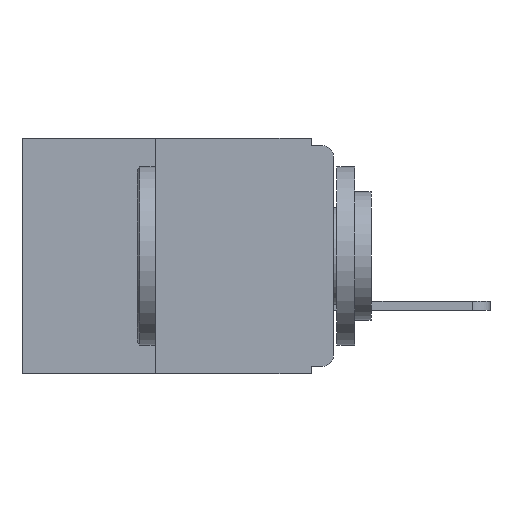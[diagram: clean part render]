
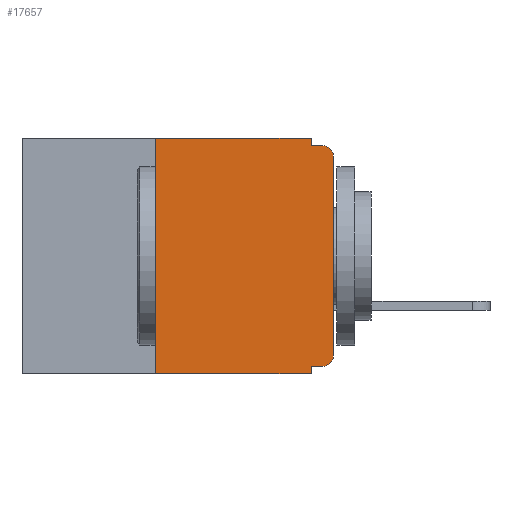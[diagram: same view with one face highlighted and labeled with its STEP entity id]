
A CAD part, left-side view. The second image highlights one B-rep face of the part: STEP entity #17657.
In plain terms, the highlighted planar face has unit normal (-1, 0, 0).
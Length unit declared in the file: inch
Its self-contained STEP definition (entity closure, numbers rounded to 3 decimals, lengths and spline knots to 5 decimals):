
#217 = CIRCLE ( 'NONE', #12686, 0.015 ) ;
#681 = FACE_OUTER_BOUND ( 'NONE', #4384, .T. ) ;
#811 = CARTESIAN_POINT ( 'NONE',  ( 0., 0., -0.32 ) ) ;
#814 = LINE ( 'NONE', #18996, #882 ) ;
#882 = VECTOR ( 'NONE', #18919, 39.37008 ) ;
#887 = VECTOR ( 'NONE', #4522, 39.37008 ) ;
#909 = LINE ( 'NONE', #4687, #887 ) ;
#1333 = DIRECTION ( 'NONE',  ( 0., 1., 0. ) ) ;
#2322 = DIRECTION ( 'NONE',  ( 0., 0., -1. ) ) ;
#2346 = VERTEX_POINT ( 'NONE', #6631 ) ;
#2395 = DIRECTION ( 'NONE',  ( -1., 0., 0. ) ) ;
#2806 = VECTOR ( 'NONE', #5126, 39.37008 ) ;
#2828 = LINE ( 'NONE', #5631, #2806 ) ;
#3031 = CARTESIAN_POINT ( 'NONE',  ( 0., 0.015, -0.305 ) ) ;
#3711 = AXIS2_PLACEMENT_3D ( 'NONE', #8074, #7900, #7869 ) ;
#3902 = LINE ( 'NONE', #811, #4075 ) ;
#3921 = LINE ( 'NONE', #19177, #4328 ) ;
#4075 = VECTOR ( 'NONE', #1333, 39.37008 ) ;
#4328 = VECTOR ( 'NONE', #19161, 39.37008 ) ;
#4384 = EDGE_LOOP ( 'NONE', ( #14196, #14783, #14862, #15110, #15358, #15587, #15747, #15940, #16102, #16426 ) ) ;
#4462 = LINE ( 'NONE', #7254, #4484 ) ;
#4479 = EDGE_CURVE ( 'NONE', #5483, #9720, #12331, .T. ) ;
#4484 = VECTOR ( 'NONE', #7374, 39.37008 ) ;
#4522 = DIRECTION ( 'NONE',  ( 0., 0., 1. ) ) ;
#4687 = CARTESIAN_POINT ( 'NONE',  ( 0., 0.25, -0.33 ) ) ;
#5126 = DIRECTION ( 'NONE',  ( 0., 0., -1. ) ) ;
#5483 = VERTEX_POINT ( 'NONE', #19361 ) ;
#5631 = CARTESIAN_POINT ( 'NONE',  ( 0., 0.031, -0.33 ) ) ;
#5644 = EDGE_CURVE ( 'NONE', #14826, #7887, #4462, .T. ) ;
#5731 = EDGE_CURVE ( 'NONE', #14055, #18590, #3902, .T. ) ;
#6120 = EDGE_CURVE ( 'NONE', #2346, #11885, #814, .T. ) ;
#6631 = CARTESIAN_POINT ( 'NONE',  ( 0., 0.25, 0. ) ) ;
#6876 = VECTOR ( 'NONE', #7334, 39.37008 ) ;
#6900 = LINE ( 'NONE', #8479, #6876 ) ;
#7254 = CARTESIAN_POINT ( 'NONE',  ( 0., 0., -0.01 ) ) ;
#7334 = DIRECTION ( 'NONE',  ( 0., 0., 1. ) ) ;
#7374 = DIRECTION ( 'NONE',  ( 0., -1., 0. ) ) ;
#7726 = CIRCLE ( 'NONE', #3711, 0.015 ) ;
#7869 = DIRECTION ( 'NONE',  ( 0., 0., -1. ) ) ;
#7876 = CARTESIAN_POINT ( 'NONE',  ( 0., 0.437, -0.33 ) ) ;
#7887 = VERTEX_POINT ( 'NONE', #19078 ) ;
#7900 = DIRECTION ( 'NONE',  ( -1., 0., 0. ) ) ;
#8074 = CARTESIAN_POINT ( 'NONE',  ( 0., 0.015, -0.025 ) ) ;
#8479 = CARTESIAN_POINT ( 'NONE',  ( 0., 0., 0. ) ) ;
#9519 = DIRECTION ( 'NONE',  ( 0., -1., 0. ) ) ;
#9720 = VERTEX_POINT ( 'NONE', #15184 ) ;
#10224 = CARTESIAN_POINT ( 'NONE',  ( 0., 0., -0.025 ) ) ;
#10346 = CARTESIAN_POINT ( 'NONE',  ( 0., 0.031, -0.32 ) ) ;
#11885 = VERTEX_POINT ( 'NONE', #12589 ) ;
#12189 = VECTOR ( 'NONE', #9519, 39.37008 ) ;
#12328 = EDGE_CURVE ( 'NONE', #5483, #2346, #909, .T. ) ;
#12331 = LINE ( 'NONE', #7876, #12189 ) ;
#12589 = CARTESIAN_POINT ( 'NONE',  ( 0., 0.031, 0. ) ) ;
#12686 = AXIS2_PLACEMENT_3D ( 'NONE', #3031, #2395, #2322 ) ;
#13381 = EDGE_CURVE ( 'NONE', #16566, #7887, #7726, .T. ) ;
#14035 = EDGE_CURVE ( 'NONE', #11885, #14826, #3921, .T. ) ;
#14055 = VERTEX_POINT ( 'NONE', #18492 ) ;
#14196 = ORIENTED_EDGE ( 'NONE', *, *, #19047, .T. ) ;
#14783 = ORIENTED_EDGE ( 'NONE', *, *, #13381, .T. ) ;
#14826 = VERTEX_POINT ( 'NONE', #18532 ) ;
#14862 = ORIENTED_EDGE ( 'NONE', *, *, #5644, .F. ) ;
#14902 = CARTESIAN_POINT ( 'NONE',  ( 0., 0., -0.305 ) ) ;
#15110 = ORIENTED_EDGE ( 'NONE', *, *, #14035, .F. ) ;
#15184 = CARTESIAN_POINT ( 'NONE',  ( 0., 0.031, -0.33 ) ) ;
#15358 = ORIENTED_EDGE ( 'NONE', *, *, #6120, .F. ) ;
#15587 = ORIENTED_EDGE ( 'NONE', *, *, #12328, .F. ) ;
#15747 = ORIENTED_EDGE ( 'NONE', *, *, #4479, .T. ) ;
#15852 = DIRECTION ( 'NONE',  ( 1., 0., 0. ) ) ;
#15940 = ORIENTED_EDGE ( 'NONE', *, *, #19401, .F. ) ;
#16035 = DIRECTION ( 'NONE',  ( 0., 0., -1. ) ) ;
#16102 = ORIENTED_EDGE ( 'NONE', *, *, #5731, .F. ) ;
#16103 = PLANE ( 'NONE',  #19146 ) ;
#16426 = ORIENTED_EDGE ( 'NONE', *, *, #19761, .T. ) ;
#16551 = CARTESIAN_POINT ( 'NONE',  ( 0., 0.437, 0. ) ) ;
#16566 = VERTEX_POINT ( 'NONE', #10224 ) ;
#17657 = ADVANCED_FACE ( 'NONE', ( #681 ), #16103, .F. ) ;
#17680 = VERTEX_POINT ( 'NONE', #14902 ) ;
#18492 = CARTESIAN_POINT ( 'NONE',  ( 0., 0.015, -0.32 ) ) ;
#18532 = CARTESIAN_POINT ( 'NONE',  ( 0., 0.031, -0.01 ) ) ;
#18590 = VERTEX_POINT ( 'NONE', #10346 ) ;
#18919 = DIRECTION ( 'NONE',  ( 0., -1., 0. ) ) ;
#18996 = CARTESIAN_POINT ( 'NONE',  ( 0., 0.437, 0. ) ) ;
#19047 = EDGE_CURVE ( 'NONE', #17680, #16566, #6900, .T. ) ;
#19078 = CARTESIAN_POINT ( 'NONE',  ( 0., 0.015, -0.01 ) ) ;
#19146 = AXIS2_PLACEMENT_3D ( 'NONE', #16551, #15852, #16035 ) ;
#19161 = DIRECTION ( 'NONE',  ( 0., 0., -1. ) ) ;
#19177 = CARTESIAN_POINT ( 'NONE',  ( 0., 0.031, 0. ) ) ;
#19361 = CARTESIAN_POINT ( 'NONE',  ( 0., 0.25, -0.33 ) ) ;
#19401 = EDGE_CURVE ( 'NONE', #18590, #9720, #2828, .T. ) ;
#19761 = EDGE_CURVE ( 'NONE', #14055, #17680, #217, .T. ) ;
